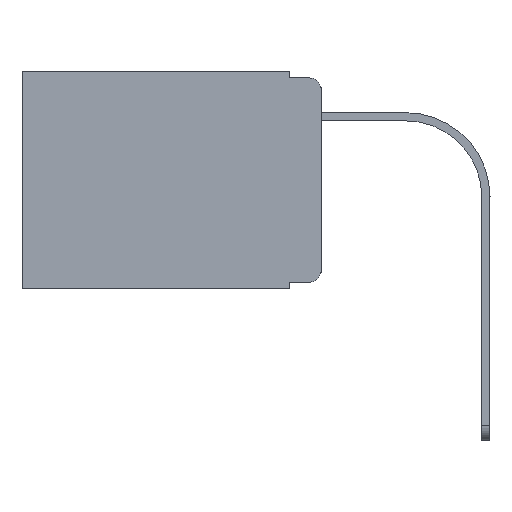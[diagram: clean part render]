
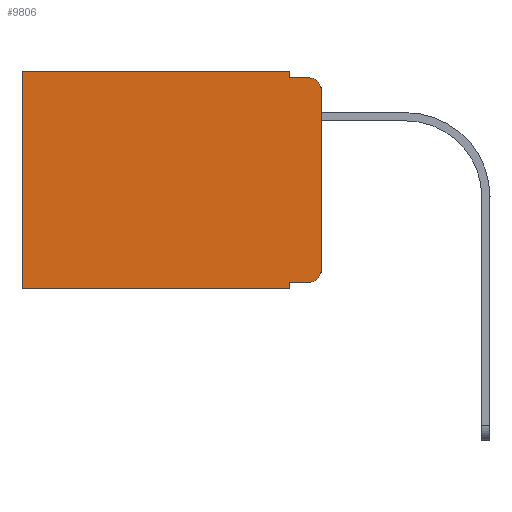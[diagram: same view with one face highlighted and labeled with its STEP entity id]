
A CAD part, left-side view. The second image highlights one B-rep face of the part: STEP entity #9806.
In plain terms, the highlighted planar face has unit normal (-1, 0, 0).
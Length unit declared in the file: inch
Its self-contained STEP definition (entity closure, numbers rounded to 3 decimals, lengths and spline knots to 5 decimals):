
#102 = AXIS2_PLACEMENT_3D ( 'NONE', #14341, #3443, #17996 ) ;
#681 = DIRECTION ( 'NONE',  ( 0., 0., -1. ) ) ;
#699 = DIRECTION ( 'NONE',  ( 0., 0., -1. ) ) ;
#765 = EDGE_CURVE ( 'NONE', #9011, #15290, #14103, .T. ) ;
#877 = EDGE_CURVE ( 'NONE', #23672, #15676, #23049, .T. ) ;
#1052 = PLANE ( 'NONE',  #11839 ) ;
#1091 = EDGE_CURVE ( 'NONE', #17632, #4706, #16454, .T. ) ;
#1508 = EDGE_CURVE ( 'NONE', #23672, #22204, #3848, .T. ) ;
#1549 = DIRECTION ( 'NONE',  ( 0., 0., -1. ) ) ;
#1558 = VECTOR ( 'NONE', #6765, 39.37008 ) ;
#2128 = ORIENTED_EDGE ( 'NONE', *, *, #765, .T. ) ;
#2377 = ORIENTED_EDGE ( 'NONE', *, *, #17460, .T. ) ;
#2646 = DIRECTION ( 'NONE',  ( 0., 0., -1. ) ) ;
#2800 = ORIENTED_EDGE ( 'NONE', *, *, #877, .F. ) ;
#2881 = CARTESIAN_POINT ( 'NONE',  ( 0.298, 0., 0. ) ) ;
#3200 = CIRCLE ( 'NONE', #102, 0.02 ) ;
#3443 = DIRECTION ( 'NONE',  ( -1., 0., 0. ) ) ;
#3451 = EDGE_CURVE ( 'NONE', #15290, #9787, #3200, .T. ) ;
#3848 = LINE ( 'NONE', #6062, #21096 ) ;
#4320 = VERTEX_POINT ( 'NONE', #17714 ) ;
#4430 = EDGE_CURVE ( 'NONE', #10780, #4320, #14990, .T. ) ;
#4706 = VERTEX_POINT ( 'NONE', #12873 ) ;
#4895 = EDGE_CURVE ( 'NONE', #15676, #4706, #22348, .T. ) ;
#5301 = CARTESIAN_POINT ( 'NONE',  ( 0.298, 0., -0.03 ) ) ;
#5593 = DIRECTION ( 'NONE',  ( -1., 0., 0. ) ) ;
#5833 = DIRECTION ( 'NONE',  ( 0., 0., -1. ) ) ;
#6062 = CARTESIAN_POINT ( 'NONE',  ( 0.298, 0., 0. ) ) ;
#6294 = AXIS2_PLACEMENT_3D ( 'NONE', #22539, #5593, #5833 ) ;
#6523 = CARTESIAN_POINT ( 'NONE',  ( 0.298, 0., 0. ) ) ;
#6765 = DIRECTION ( 'NONE',  ( 0., -1., 0. ) ) ;
#8781 = CARTESIAN_POINT ( 'NONE',  ( 0.298, 0.051, 0. ) ) ;
#9011 = VERTEX_POINT ( 'NONE', #20690 ) ;
#9437 = CARTESIAN_POINT ( 'NONE',  ( 0.298, 0.051, -0.01 ) ) ;
#9497 = DIRECTION ( 'NONE',  ( 0., 1., 0. ) ) ;
#9787 = VERTEX_POINT ( 'NONE', #15500 ) ;
#9806 = ADVANCED_FACE ( 'NONE', ( #17447 ), #1052, .F. ) ;
#9917 = DIRECTION ( 'NONE',  ( 0., 0., -1. ) ) ;
#10049 = EDGE_LOOP ( 'NONE', ( #17660, #20893, #11084, #2800, #14440, #2377, #19832, #23419, #2128, #12857 ) ) ;
#10531 = VECTOR ( 'NONE', #681, 39.37008 ) ;
#10728 = VECTOR ( 'NONE', #17021, 39.37008 ) ;
#10780 = VERTEX_POINT ( 'NONE', #22173 ) ;
#11084 = ORIENTED_EDGE ( 'NONE', *, *, #4895, .F. ) ;
#11238 = VECTOR ( 'NONE', #1549, 39.37008 ) ;
#11459 = EDGE_CURVE ( 'NONE', #17632, #9787, #19118, .T. ) ;
#11839 = AXIS2_PLACEMENT_3D ( 'NONE', #2881, #19379, #2646 ) ;
#12684 = VECTOR ( 'NONE', #21035, 39.37008 ) ;
#12857 = ORIENTED_EDGE ( 'NONE', *, *, #3451, .T. ) ;
#12873 = CARTESIAN_POINT ( 'NONE',  ( 0.298, 0.02, -0.01 ) ) ;
#13799 = CARTESIAN_POINT ( 'NONE',  ( 0.298, 0.473, 0. ) ) ;
#14103 = LINE ( 'NONE', #21727, #1558 ) ;
#14341 = CARTESIAN_POINT ( 'NONE',  ( 0.298, 0.02, -0.313 ) ) ;
#14440 = ORIENTED_EDGE ( 'NONE', *, *, #1508, .T. ) ;
#14496 = VECTOR ( 'NONE', #9917, 39.37008 ) ;
#14961 = CARTESIAN_POINT ( 'NONE',  ( 0.298, 0.051, -0.01 ) ) ;
#14990 = LINE ( 'NONE', #22493, #12684 ) ;
#15290 = VERTEX_POINT ( 'NONE', #20577 ) ;
#15500 = CARTESIAN_POINT ( 'NONE',  ( 0.298, 0., -0.313 ) ) ;
#15676 = VERTEX_POINT ( 'NONE', #9437 ) ;
#16182 = VECTOR ( 'NONE', #699, 39.37008 ) ;
#16454 = CIRCLE ( 'NONE', #6294, 0.02 ) ;
#16737 = CARTESIAN_POINT ( 'NONE',  ( 0.298, 0.473, 0. ) ) ;
#17021 = DIRECTION ( 'NONE',  ( 0., -1., 0. ) ) ;
#17447 = FACE_OUTER_BOUND ( 'NONE', #10049, .T. ) ;
#17460 = EDGE_CURVE ( 'NONE', #22204, #4320, #19140, .T. ) ;
#17632 = VERTEX_POINT ( 'NONE', #5301 ) ;
#17660 = ORIENTED_EDGE ( 'NONE', *, *, #11459, .F. ) ;
#17714 = CARTESIAN_POINT ( 'NONE',  ( 0.298, 0.473, -0.343 ) ) ;
#17996 = DIRECTION ( 'NONE',  ( 0., 0., -1. ) ) ;
#18063 = LINE ( 'NONE', #8781, #11238 ) ;
#19063 = CARTESIAN_POINT ( 'NONE',  ( 0.298, 0.051, 0. ) ) ;
#19118 = LINE ( 'NONE', #6523, #10531 ) ;
#19140 = LINE ( 'NONE', #13799, #16182 ) ;
#19379 = DIRECTION ( 'NONE',  ( 1., 0., 0. ) ) ;
#19832 = ORIENTED_EDGE ( 'NONE', *, *, #4430, .F. ) ;
#20577 = CARTESIAN_POINT ( 'NONE',  ( 0.298, 0.02, -0.333 ) ) ;
#20690 = CARTESIAN_POINT ( 'NONE',  ( 0.298, 0.051, -0.333 ) ) ;
#20893 = ORIENTED_EDGE ( 'NONE', *, *, #1091, .T. ) ;
#21035 = DIRECTION ( 'NONE',  ( 0., 1., 0. ) ) ;
#21096 = VECTOR ( 'NONE', #9497, 39.37008 ) ;
#21390 = EDGE_CURVE ( 'NONE', #9011, #10780, #18063, .T. ) ;
#21727 = CARTESIAN_POINT ( 'NONE',  ( 0.298, 0.051, -0.333 ) ) ;
#22173 = CARTESIAN_POINT ( 'NONE',  ( 0.298, 0.051, -0.343 ) ) ;
#22204 = VERTEX_POINT ( 'NONE', #16737 ) ;
#22348 = LINE ( 'NONE', #14961, #10728 ) ;
#22493 = CARTESIAN_POINT ( 'NONE',  ( 0.298, 0., -0.343 ) ) ;
#22539 = CARTESIAN_POINT ( 'NONE',  ( 0.298, 0.02, -0.03 ) ) ;
#23049 = LINE ( 'NONE', #19063, #14496 ) ;
#23419 = ORIENTED_EDGE ( 'NONE', *, *, #21390, .F. ) ;
#23672 = VERTEX_POINT ( 'NONE', #24051 ) ;
#24051 = CARTESIAN_POINT ( 'NONE',  ( 0.298, 0.051, 0. ) ) ;
